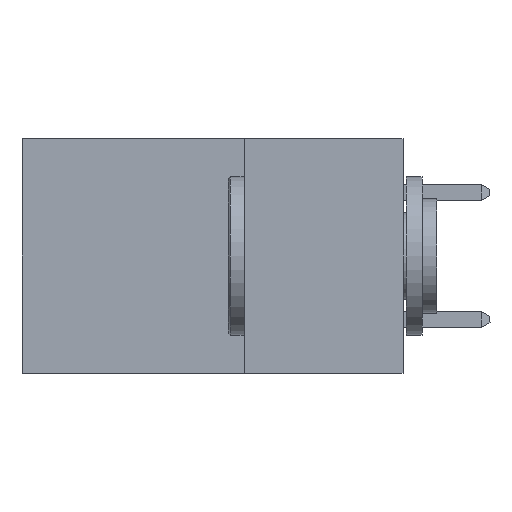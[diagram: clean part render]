
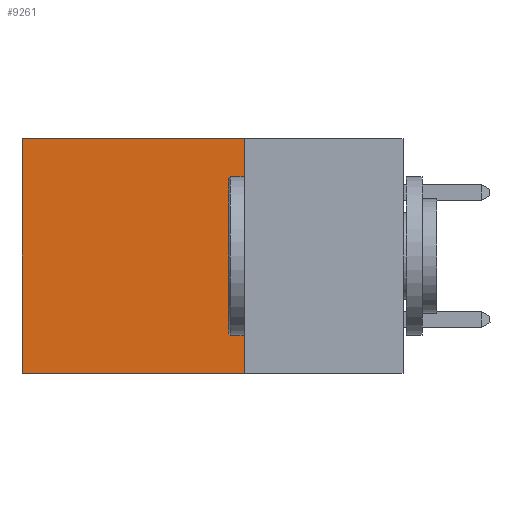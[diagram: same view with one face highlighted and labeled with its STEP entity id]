
A CAD part, left-side view. The second image highlights one B-rep face of the part: STEP entity #9261.
In plain terms, the highlighted planar face has unit normal (-1, 0, 0).
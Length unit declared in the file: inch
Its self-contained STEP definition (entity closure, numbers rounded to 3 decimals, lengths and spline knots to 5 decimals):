
#437 = DIRECTION ( 'NONE',  ( 0., 1., 0. ) ) ;
#739 = ORIENTED_EDGE ( 'NONE', *, *, #14926, .T. ) ;
#1283 = DIRECTION ( 'NONE',  ( 0., 0., -1. ) ) ;
#1324 = VECTOR ( 'NONE', #437, 39.37008 ) ;
#1620 = DIRECTION ( 'NONE',  ( 0., 1., 0. ) ) ;
#1932 = PLANE ( 'NONE',  #14520 ) ;
#2719 = CARTESIAN_POINT ( 'NONE',  ( 0.2875, 0.6, 0. ) ) ;
#3044 = LINE ( 'NONE', #7843, #1324 ) ;
#3798 = VERTEX_POINT ( 'NONE', #2719 ) ;
#3934 = DIRECTION ( 'NONE',  ( 0., 0., -1. ) ) ;
#4191 = ORIENTED_EDGE ( 'NONE', *, *, #5436, .F. ) ;
#5381 = CARTESIAN_POINT ( 'NONE',  ( 0.2875, 0.25, -0.37 ) ) ;
#5436 = EDGE_CURVE ( 'NONE', #12674, #5789, #6385, .T. ) ;
#5469 = DIRECTION ( 'NONE',  ( 0., 0., -1. ) ) ;
#5789 = VERTEX_POINT ( 'NONE', #13245 ) ;
#6385 = LINE ( 'NONE', #7471, #13739 ) ;
#6518 = ORIENTED_EDGE ( 'NONE', *, *, #10716, .F. ) ;
#7471 = CARTESIAN_POINT ( 'NONE',  ( 0.2875, 0.25, 0. ) ) ;
#7843 = CARTESIAN_POINT ( 'NONE',  ( 0.2875, 0.25, 0. ) ) ;
#8164 = VERTEX_POINT ( 'NONE', #15158 ) ;
#9261 = ADVANCED_FACE ( 'NONE', ( #11216 ), #1932, .F. ) ;
#9502 = LINE ( 'NONE', #9981, #14334 ) ;
#9864 = EDGE_LOOP ( 'NONE', ( #739, #6518, #4191, #10839 ) ) ;
#9981 = CARTESIAN_POINT ( 'NONE',  ( 0.2875, 0.6, 0. ) ) ;
#10617 = VECTOR ( 'NONE', #1620, 39.37008 ) ;
#10644 = DIRECTION ( 'NONE',  ( 1., 0., 0. ) ) ;
#10716 = EDGE_CURVE ( 'NONE', #5789, #8164, #16064, .T. ) ;
#10839 = ORIENTED_EDGE ( 'NONE', *, *, #15687, .T. ) ;
#11216 = FACE_OUTER_BOUND ( 'NONE', #9864, .T. ) ;
#12674 = VERTEX_POINT ( 'NONE', #13117 ) ;
#12922 = CARTESIAN_POINT ( 'NONE',  ( 0.2875, 0.25, 0. ) ) ;
#13117 = CARTESIAN_POINT ( 'NONE',  ( 0.2875, 0.25, 0. ) ) ;
#13245 = CARTESIAN_POINT ( 'NONE',  ( 0.2875, 0.25, -0.37 ) ) ;
#13739 = VECTOR ( 'NONE', #1283, 39.37008 ) ;
#14334 = VECTOR ( 'NONE', #3934, 39.37008 ) ;
#14520 = AXIS2_PLACEMENT_3D ( 'NONE', #12922, #10644, #5469 ) ;
#14926 = EDGE_CURVE ( 'NONE', #3798, #8164, #9502, .T. ) ;
#15158 = CARTESIAN_POINT ( 'NONE',  ( 0.2875, 0.6, -0.37 ) ) ;
#15687 = EDGE_CURVE ( 'NONE', #12674, #3798, #3044, .T. ) ;
#16064 = LINE ( 'NONE', #5381, #10617 ) ;
